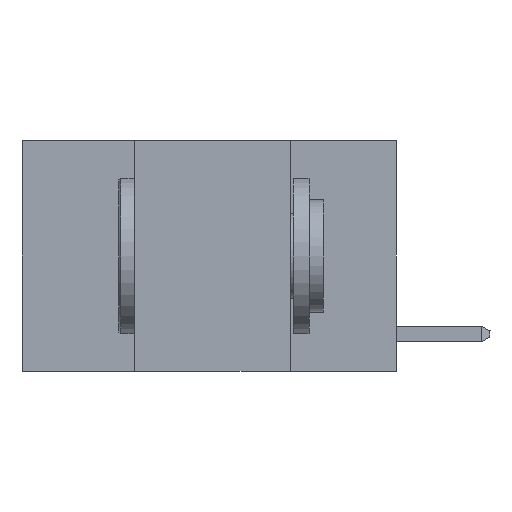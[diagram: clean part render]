
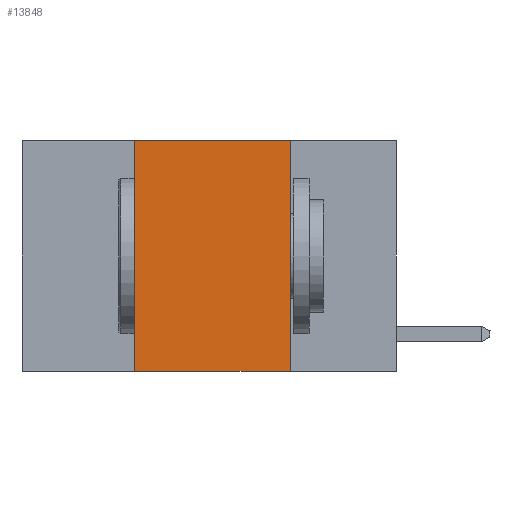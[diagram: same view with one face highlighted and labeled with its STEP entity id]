
A CAD part, left-side view. The second image highlights one B-rep face of the part: STEP entity #13848.
In plain terms, the highlighted planar face has unit normal (-1, 0, 0).
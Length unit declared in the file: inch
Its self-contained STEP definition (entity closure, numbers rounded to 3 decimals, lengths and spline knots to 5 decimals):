
#908 = LINE ( 'NONE', #15724, #7904 ) ;
#1678 = CARTESIAN_POINT ( 'NONE',  ( 0., 0.42, -0.37 ) ) ;
#1984 = LINE ( 'NONE', #8146, #16750 ) ;
#2072 = EDGE_CURVE ( 'NONE', #12385, #4760, #8657, .T. ) ;
#2707 = CARTESIAN_POINT ( 'NONE',  ( 0., 0.42, 0. ) ) ;
#4172 = CARTESIAN_POINT ( 'NONE',  ( 0., 0.6, 0. ) ) ;
#4760 = VERTEX_POINT ( 'NONE', #2707 ) ;
#4796 = ORIENTED_EDGE ( 'NONE', *, *, #12034, .F. ) ;
#4913 = CARTESIAN_POINT ( 'NONE',  ( 0., 0.17, -0.37 ) ) ;
#5123 = AXIS2_PLACEMENT_3D ( 'NONE', #4172, #19438, #6039 ) ;
#5375 = DIRECTION ( 'NONE',  ( 0., -1., 0. ) ) ;
#6039 = DIRECTION ( 'NONE',  ( 0., 0., -1. ) ) ;
#6495 = LINE ( 'NONE', #6605, #12160 ) ;
#6605 = CARTESIAN_POINT ( 'NONE',  ( 0., 0.6, -0.37 ) ) ;
#7074 = DIRECTION ( 'NONE',  ( 0., 0., 1. ) ) ;
#7172 = CARTESIAN_POINT ( 'NONE',  ( 0., 0.42, 0. ) ) ;
#7867 = VERTEX_POINT ( 'NONE', #4913 ) ;
#7904 = VECTOR ( 'NONE', #5375, 39.37008 ) ;
#8146 = CARTESIAN_POINT ( 'NONE',  ( 0., 0.17, 0. ) ) ;
#8657 = LINE ( 'NONE', #7172, #11861 ) ;
#8751 = PLANE ( 'NONE',  #5123 ) ;
#9306 = ORIENTED_EDGE ( 'NONE', *, *, #11405, .T. ) ;
#10851 = CARTESIAN_POINT ( 'NONE',  ( 0., 0.17, 0. ) ) ;
#11405 = EDGE_CURVE ( 'NONE', #12385, #7867, #6495, .T. ) ;
#11445 = VERTEX_POINT ( 'NONE', #10851 ) ;
#11517 = EDGE_LOOP ( 'NONE', ( #14835, #4796, #16768, #9306 ) ) ;
#11861 = VECTOR ( 'NONE', #7074, 39.37008 ) ;
#12034 = EDGE_CURVE ( 'NONE', #4760, #11445, #908, .T. ) ;
#12160 = VECTOR ( 'NONE', #16929, 39.37008 ) ;
#12385 = VERTEX_POINT ( 'NONE', #1678 ) ;
#13593 = EDGE_CURVE ( 'NONE', #11445, #7867, #1984, .T. ) ;
#13848 = ADVANCED_FACE ( 'NONE', ( #15111 ), #8751, .F. ) ;
#14835 = ORIENTED_EDGE ( 'NONE', *, *, #13593, .F. ) ;
#15111 = FACE_OUTER_BOUND ( 'NONE', #11517, .T. ) ;
#15724 = CARTESIAN_POINT ( 'NONE',  ( 0., 0.6, 0. ) ) ;
#16750 = VECTOR ( 'NONE', #16781, 39.37008 ) ;
#16768 = ORIENTED_EDGE ( 'NONE', *, *, #2072, .F. ) ;
#16781 = DIRECTION ( 'NONE',  ( 0., 0., -1. ) ) ;
#16929 = DIRECTION ( 'NONE',  ( 0., -1., 0. ) ) ;
#19438 = DIRECTION ( 'NONE',  ( 1., 0., 0. ) ) ;
